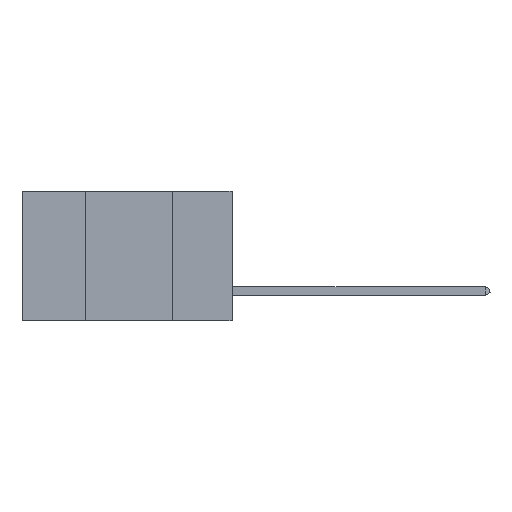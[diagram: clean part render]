
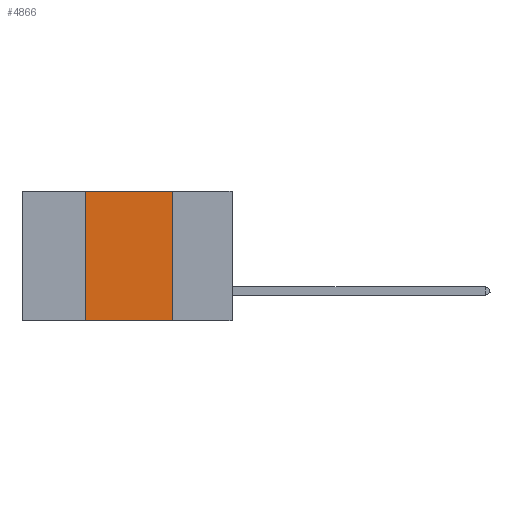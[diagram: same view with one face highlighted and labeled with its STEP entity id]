
A CAD part, left-side view. The second image highlights one B-rep face of the part: STEP entity #4866.
In plain terms, the highlighted planar face has unit normal (-1, 0, 0).
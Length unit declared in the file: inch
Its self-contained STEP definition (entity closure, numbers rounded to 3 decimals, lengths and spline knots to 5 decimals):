
#113 = EDGE_LOOP ( 'NONE', ( #11195, #3521, #7125, #3541 ) ) ;
#148 = CARTESIAN_POINT ( 'NONE',  ( 0., 0.6, 0. ) ) ;
#766 = CARTESIAN_POINT ( 'NONE',  ( 0., 0.6, 0. ) ) ;
#1067 = EDGE_CURVE ( 'NONE', #4427, #6930, #4289, .T. ) ;
#1085 = CARTESIAN_POINT ( 'NONE',  ( 0., 0.17, 0. ) ) ;
#1479 = FACE_OUTER_BOUND ( 'NONE', #113, .T. ) ;
#1607 = DIRECTION ( 'NONE',  ( 0., 0., 1. ) ) ;
#1840 = CARTESIAN_POINT ( 'NONE',  ( 0., 0.42, -0.37 ) ) ;
#1905 = PLANE ( 'NONE',  #4817 ) ;
#2163 = LINE ( 'NONE', #6267, #4374 ) ;
#2400 = DIRECTION ( 'NONE',  ( 0., -1., 0. ) ) ;
#2588 = VERTEX_POINT ( 'NONE', #9184 ) ;
#3521 = ORIENTED_EDGE ( 'NONE', *, *, #8383, .F. ) ;
#3541 = ORIENTED_EDGE ( 'NONE', *, *, #9624, .T. ) ;
#3888 = LINE ( 'NONE', #4277, #11939 ) ;
#4277 = CARTESIAN_POINT ( 'NONE',  ( 0., 0.17, 0. ) ) ;
#4289 = LINE ( 'NONE', #12107, #12198 ) ;
#4374 = VECTOR ( 'NONE', #2400, 39.37008 ) ;
#4427 = VERTEX_POINT ( 'NONE', #1840 ) ;
#4611 = CARTESIAN_POINT ( 'NONE',  ( 0., 0.42, 0. ) ) ;
#4817 = AXIS2_PLACEMENT_3D ( 'NONE', #766, #9516, #5519 ) ;
#4866 = ADVANCED_FACE ( 'NONE', ( #1479 ), #1905, .F. ) ;
#5382 = LINE ( 'NONE', #148, #11053 ) ;
#5519 = DIRECTION ( 'NONE',  ( 0., 0., -1. ) ) ;
#5899 = DIRECTION ( 'NONE',  ( 0., -1., 0. ) ) ;
#6129 = DIRECTION ( 'NONE',  ( 0., 0., -1. ) ) ;
#6267 = CARTESIAN_POINT ( 'NONE',  ( 0., 0.6, -0.37 ) ) ;
#6930 = VERTEX_POINT ( 'NONE', #4611 ) ;
#7125 = ORIENTED_EDGE ( 'NONE', *, *, #1067, .F. ) ;
#8383 = EDGE_CURVE ( 'NONE', #6930, #11079, #5382, .T. ) ;
#9184 = CARTESIAN_POINT ( 'NONE',  ( 0., 0.17, -0.37 ) ) ;
#9516 = DIRECTION ( 'NONE',  ( 1., 0., 0. ) ) ;
#9624 = EDGE_CURVE ( 'NONE', #4427, #2588, #2163, .T. ) ;
#11053 = VECTOR ( 'NONE', #5899, 39.37008 ) ;
#11079 = VERTEX_POINT ( 'NONE', #1085 ) ;
#11195 = ORIENTED_EDGE ( 'NONE', *, *, #11340, .F. ) ;
#11340 = EDGE_CURVE ( 'NONE', #11079, #2588, #3888, .T. ) ;
#11939 = VECTOR ( 'NONE', #6129, 39.37008 ) ;
#12107 = CARTESIAN_POINT ( 'NONE',  ( 0., 0.42, 0. ) ) ;
#12198 = VECTOR ( 'NONE', #1607, 39.37008 ) ;
